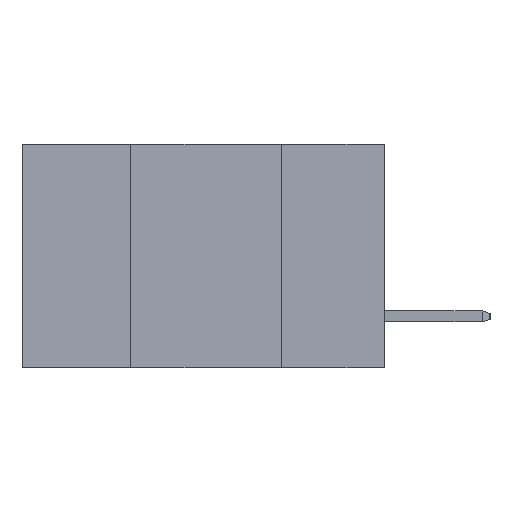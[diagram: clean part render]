
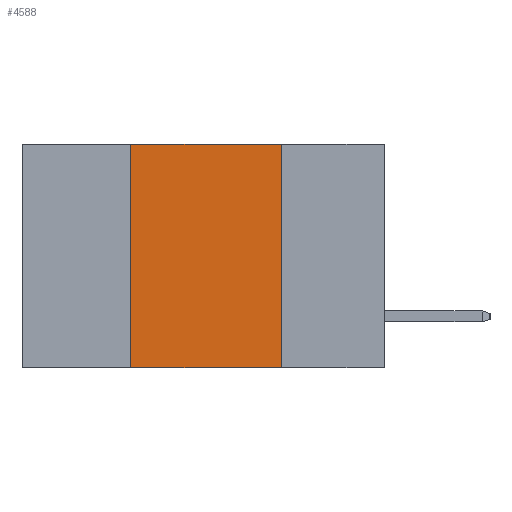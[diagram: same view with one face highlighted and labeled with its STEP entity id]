
A CAD part, left-side view. The second image highlights one B-rep face of the part: STEP entity #4588.
In plain terms, the highlighted planar face has unit normal (-1, 0, 0).
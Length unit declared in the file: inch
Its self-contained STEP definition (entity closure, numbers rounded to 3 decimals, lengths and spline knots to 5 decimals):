
#45 = EDGE_LOOP ( 'NONE', ( #12811, #15854, #9622, #8786 ) ) ;
#2403 = CARTESIAN_POINT ( 'NONE',  ( 0., 0.6, -0.37 ) ) ;
#2760 = DIRECTION ( 'NONE',  ( 0., -1., 0. ) ) ;
#4220 = EDGE_CURVE ( 'NONE', #7948, #11136, #9984, .T. ) ;
#4588 = ADVANCED_FACE ( 'NONE', ( #16373 ), #11012, .F. ) ;
#5099 = EDGE_CURVE ( 'NONE', #11136, #20378, #9702, .T. ) ;
#7563 = VECTOR ( 'NONE', #8324, 39.37008 ) ;
#7948 = VERTEX_POINT ( 'NONE', #20520 ) ;
#8324 = DIRECTION ( 'NONE',  ( 0., 0., 1. ) ) ;
#8786 = ORIENTED_EDGE ( 'NONE', *, *, #13729, .T. ) ;
#9385 = DIRECTION ( 'NONE',  ( 0., -1., 0. ) ) ;
#9426 = VECTOR ( 'NONE', #9385, 39.37008 ) ;
#9622 = ORIENTED_EDGE ( 'NONE', *, *, #21731, .F. ) ;
#9702 = LINE ( 'NONE', #11030, #22969 ) ;
#9845 = CARTESIAN_POINT ( 'NONE',  ( 0., 0.6, 0. ) ) ;
#9982 = CARTESIAN_POINT ( 'NONE',  ( 0., 0.42, -0.37 ) ) ;
#9984 = LINE ( 'NONE', #9845, #9426 ) ;
#10135 = VERTEX_POINT ( 'NONE', #9982 ) ;
#10329 = DIRECTION ( 'NONE',  ( 1., 0., 0. ) ) ;
#10361 = DIRECTION ( 'NONE',  ( 0., 0., -1. ) ) ;
#10559 = CARTESIAN_POINT ( 'NONE',  ( 0., 0.6, 0. ) ) ;
#11012 = PLANE ( 'NONE',  #21333 ) ;
#11030 = CARTESIAN_POINT ( 'NONE',  ( 0., 0.17, -0.37 ) ) ;
#11088 = DIRECTION ( 'NONE',  ( 0., 0., -1. ) ) ;
#11136 = VERTEX_POINT ( 'NONE', #19215 ) ;
#11817 = CARTESIAN_POINT ( 'NONE',  ( 0., 0.42, -0.37 ) ) ;
#12811 = ORIENTED_EDGE ( 'NONE', *, *, #5099, .F. ) ;
#12952 = VECTOR ( 'NONE', #2760, 39.37008 ) ;
#13513 = LINE ( 'NONE', #2403, #12952 ) ;
#13729 = EDGE_CURVE ( 'NONE', #10135, #20378, #13513, .T. ) ;
#15854 = ORIENTED_EDGE ( 'NONE', *, *, #4220, .F. ) ;
#16373 = FACE_OUTER_BOUND ( 'NONE', #45, .T. ) ;
#18579 = CARTESIAN_POINT ( 'NONE',  ( 0., 0.17, -0.37 ) ) ;
#19215 = CARTESIAN_POINT ( 'NONE',  ( 0., 0.17, 0. ) ) ;
#20378 = VERTEX_POINT ( 'NONE', #18579 ) ;
#20520 = CARTESIAN_POINT ( 'NONE',  ( 0., 0.42, 0. ) ) ;
#21333 = AXIS2_PLACEMENT_3D ( 'NONE', #10559, #10329, #10361 ) ;
#21731 = EDGE_CURVE ( 'NONE', #10135, #7948, #22587, .T. ) ;
#22587 = LINE ( 'NONE', #11817, #7563 ) ;
#22969 = VECTOR ( 'NONE', #11088, 39.37008 ) ;
